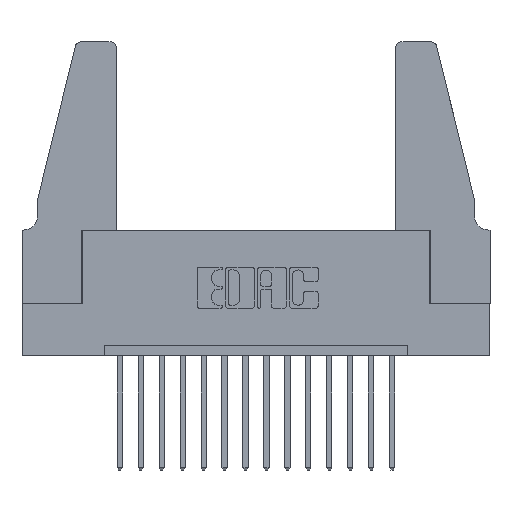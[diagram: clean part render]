
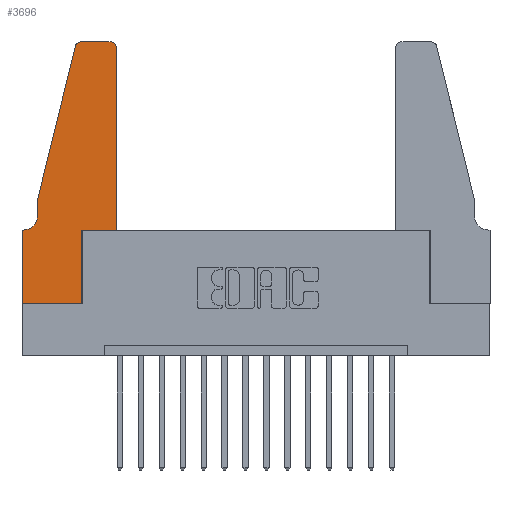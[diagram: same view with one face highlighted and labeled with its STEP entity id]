
A CAD part, top view. The second image highlights one B-rep face of the part: STEP entity #3696.
In plain terms, the highlighted planar face has unit normal (0, 0, 1).
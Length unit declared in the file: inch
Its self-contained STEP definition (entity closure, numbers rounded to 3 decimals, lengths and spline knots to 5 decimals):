
#92 = EDGE_CURVE ( 'NONE', #5823, #6624, #14274, .T. ) ;
#190 = CARTESIAN_POINT ( 'NONE',  ( 0., 0.35, 0.37 ) ) ;
#304 = VECTOR ( 'NONE', #11447, 39.37008 ) ;
#386 = DIRECTION ( 'NONE',  ( 0., 0., 1. ) ) ;
#530 = CARTESIAN_POINT ( 'NONE',  ( 0.2605, 1.25, 0.37 ) ) ;
#544 = AXIS2_PLACEMENT_3D ( 'NONE', #3726, #4931, #3834 ) ;
#577 = CARTESIAN_POINT ( 'NONE',  ( 0.0755, 0.5, 0.37 ) ) ;
#580 = CARTESIAN_POINT ( 'NONE',  ( 0.2865, 0., 0.37 ) ) ;
#607 = FACE_OUTER_BOUND ( 'NONE', #6382, .T. ) ;
#1301 = ORIENTED_EDGE ( 'NONE', *, *, #6665, .T. ) ;
#1539 = CARTESIAN_POINT ( 'NONE',  ( 0., 0.35, 0.37 ) ) ;
#1875 = DIRECTION ( 'NONE',  ( -0.239, -0.971, 0. ) ) ;
#1985 = LINE ( 'NONE', #12626, #15111 ) ;
#2361 = CIRCLE ( 'NONE', #544, 0.07 ) ;
#2407 = LINE ( 'NONE', #7195, #9942 ) ;
#2463 = EDGE_CURVE ( 'NONE', #6460, #8451, #11011, .T. ) ;
#2497 = ORIENTED_EDGE ( 'NONE', *, *, #3154, .T. ) ;
#2594 = CARTESIAN_POINT ( 'NONE',  ( 0.2865, 0.35, 0.37 ) ) ;
#2748 = CARTESIAN_POINT ( 'NONE',  ( 0.284, 1.22, 0.37 ) ) ;
#2861 = DIRECTION ( 'NONE',  ( 1., 0., 0. ) ) ;
#3000 = ORIENTED_EDGE ( 'NONE', *, *, #3569, .T. ) ;
#3027 = ORIENTED_EDGE ( 'NONE', *, *, #7563, .T. ) ;
#3154 = EDGE_CURVE ( 'NONE', #6624, #3175, #6308, .T. ) ;
#3175 = VERTEX_POINT ( 'NONE', #7090 ) ;
#3436 = ORIENTED_EDGE ( 'NONE', *, *, #12675, .T. ) ;
#3569 = EDGE_CURVE ( 'NONE', #11050, #6966, #1985, .T. ) ;
#3696 = ADVANCED_FACE ( 'NONE', ( #607 ), #8003, .T. ) ;
#3697 = VECTOR ( 'NONE', #1875, 39.37008 ) ;
#3726 = CARTESIAN_POINT ( 'NONE',  ( 0.0055, 0.42, 0.37 ) ) ;
#3834 = DIRECTION ( 'NONE',  ( -1., 0., 0. ) ) ;
#3959 = ORIENTED_EDGE ( 'NONE', *, *, #4845, .T. ) ;
#4392 = VERTEX_POINT ( 'NONE', #7995 ) ;
#4422 = ORIENTED_EDGE ( 'NONE', *, *, #92, .T. ) ;
#4586 = DIRECTION ( 'NONE',  ( 0., 1., 0. ) ) ;
#4790 = AXIS2_PLACEMENT_3D ( 'NONE', #1539, #386, #9225 ) ;
#4803 = LINE ( 'NONE', #15620, #11148 ) ;
#4845 = EDGE_CURVE ( 'NONE', #9748, #5823, #2407, .T. ) ;
#4849 = ORIENTED_EDGE ( 'NONE', *, *, #14263, .T. ) ;
#4851 = DIRECTION ( 'NONE',  ( -1., 0., 0. ) ) ;
#4931 = DIRECTION ( 'NONE',  ( 0., 0., -1. ) ) ;
#4937 = ORIENTED_EDGE ( 'NONE', *, *, #5776, .T. ) ;
#5243 = VECTOR ( 'NONE', #9968, 39.37008 ) ;
#5289 = DIRECTION ( 'NONE',  ( 0., 0., 1. ) ) ;
#5431 = DIRECTION ( 'NONE',  ( 1., 0., 0. ) ) ;
#5483 = CARTESIAN_POINT ( 'NONE',  ( 0.4205, 1.25, 0.37 ) ) ;
#5776 = EDGE_CURVE ( 'NONE', #6966, #9748, #15799, .T. ) ;
#5823 = VERTEX_POINT ( 'NONE', #10409 ) ;
#5833 = CIRCLE ( 'NONE', #16162, 0.03 ) ;
#6308 = LINE ( 'NONE', #530, #8854 ) ;
#6382 = EDGE_LOOP ( 'NONE', ( #2497, #4849, #11691, #14016, #16435, #3027, #3436, #1301, #3000, #4937, #3959, #4422 ) ) ;
#6460 = VERTEX_POINT ( 'NONE', #15460 ) ;
#6624 = VERTEX_POINT ( 'NONE', #5483 ) ;
#6665 = EDGE_CURVE ( 'NONE', #8923, #11050, #4803, .T. ) ;
#6966 = VERTEX_POINT ( 'NONE', #2594 ) ;
#7090 = CARTESIAN_POINT ( 'NONE',  ( 0.284, 1.25, 0.37 ) ) ;
#7195 = CARTESIAN_POINT ( 'NONE',  ( 0.4505, 0.35, 0.37 ) ) ;
#7563 = EDGE_CURVE ( 'NONE', #10027, #15914, #9719, .T. ) ;
#7995 = CARTESIAN_POINT ( 'NONE',  ( 0.0755, 0.42, 0.37 ) ) ;
#8003 = PLANE ( 'NONE',  #4790 ) ;
#8053 = LINE ( 'NONE', #8780, #304 ) ;
#8451 = VERTEX_POINT ( 'NONE', #13180 ) ;
#8780 = CARTESIAN_POINT ( 'NONE',  ( 0.0755, 0.5, 0.37 ) ) ;
#8785 = CARTESIAN_POINT ( 'NONE',  ( 0.4505, 0.35, 0.37 ) ) ;
#8854 = VECTOR ( 'NONE', #11858, 39.37008 ) ;
#8923 = VERTEX_POINT ( 'NONE', #12379 ) ;
#9211 = AXIS2_PLACEMENT_3D ( 'NONE', #10541, #11663, #2861 ) ;
#9225 = DIRECTION ( 'NONE',  ( 1., 0., 0. ) ) ;
#9719 = LINE ( 'NONE', #11170, #15109 ) ;
#9748 = VERTEX_POINT ( 'NONE', #11725 ) ;
#9942 = VECTOR ( 'NONE', #4586, 39.37008 ) ;
#9968 = DIRECTION ( 'NONE',  ( 1., 0., 0. ) ) ;
#10027 = VERTEX_POINT ( 'NONE', #14204 ) ;
#10259 = EDGE_CURVE ( 'NONE', #8451, #4392, #8053, .T. ) ;
#10409 = CARTESIAN_POINT ( 'NONE',  ( 0.4505, 1.22, 0.37 ) ) ;
#10541 = CARTESIAN_POINT ( 'NONE',  ( 0.4205, 1.22, 0.37 ) ) ;
#11011 = LINE ( 'NONE', #577, #3697 ) ;
#11050 = VERTEX_POINT ( 'NONE', #580 ) ;
#11148 = VECTOR ( 'NONE', #5431, 39.37008 ) ;
#11170 = CARTESIAN_POINT ( 'NONE',  ( 0.0755, 0.35, 0.37 ) ) ;
#11447 = DIRECTION ( 'NONE',  ( 0., -1., 0. ) ) ;
#11547 = DIRECTION ( 'NONE',  ( 1., 0., 0. ) ) ;
#11663 = DIRECTION ( 'NONE',  ( 0., 0., 1. ) ) ;
#11691 = ORIENTED_EDGE ( 'NONE', *, *, #2463, .T. ) ;
#11725 = CARTESIAN_POINT ( 'NONE',  ( 0.4505, 0.35, 0.37 ) ) ;
#11858 = DIRECTION ( 'NONE',  ( -1., 0., 0. ) ) ;
#12379 = CARTESIAN_POINT ( 'NONE',  ( 0., 0., 0.37 ) ) ;
#12454 = EDGE_CURVE ( 'NONE', #4392, #10027, #2361, .T. ) ;
#12626 = CARTESIAN_POINT ( 'NONE',  ( 0.2865, 0.35, 0.37 ) ) ;
#12675 = EDGE_CURVE ( 'NONE', #15914, #8923, #15670, .T. ) ;
#13063 = VECTOR ( 'NONE', #14357, 39.37008 ) ;
#13086 = CARTESIAN_POINT ( 'NONE',  ( 0., 0., 0.37 ) ) ;
#13180 = CARTESIAN_POINT ( 'NONE',  ( 0.0755, 0.5, 0.37 ) ) ;
#14016 = ORIENTED_EDGE ( 'NONE', *, *, #10259, .T. ) ;
#14204 = CARTESIAN_POINT ( 'NONE',  ( 0.0055, 0.35, 0.37 ) ) ;
#14263 = EDGE_CURVE ( 'NONE', #3175, #6460, #5833, .T. ) ;
#14274 = CIRCLE ( 'NONE', #9211, 0.03 ) ;
#14357 = DIRECTION ( 'NONE',  ( 0., -1., 0. ) ) ;
#15109 = VECTOR ( 'NONE', #4851, 39.37008 ) ;
#15111 = VECTOR ( 'NONE', #15445, 39.37008 ) ;
#15445 = DIRECTION ( 'NONE',  ( 0., 1., 0. ) ) ;
#15460 = CARTESIAN_POINT ( 'NONE',  ( 0.25487, 1.22718, 0.37 ) ) ;
#15620 = CARTESIAN_POINT ( 'NONE',  ( 0., 0., 0.37 ) ) ;
#15670 = LINE ( 'NONE', #13086, #13063 ) ;
#15799 = LINE ( 'NONE', #8785, #5243 ) ;
#15914 = VERTEX_POINT ( 'NONE', #190 ) ;
#16162 = AXIS2_PLACEMENT_3D ( 'NONE', #2748, #5289, #11547 ) ;
#16435 = ORIENTED_EDGE ( 'NONE', *, *, #12454, .T. ) ;
